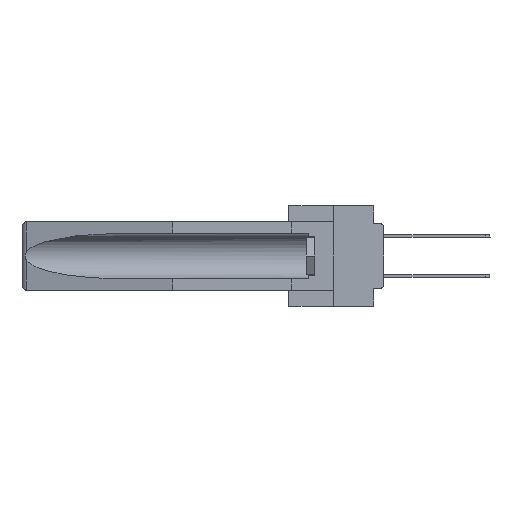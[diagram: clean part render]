
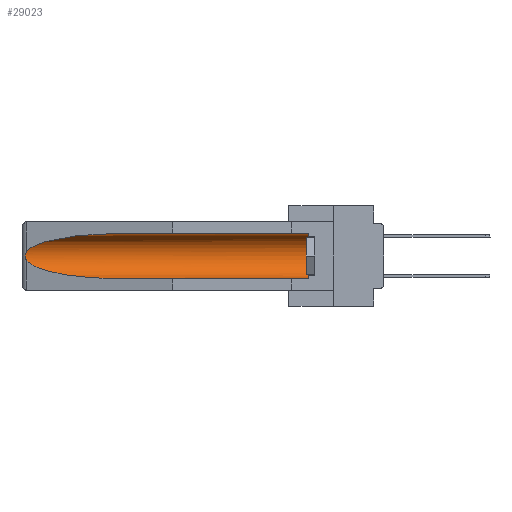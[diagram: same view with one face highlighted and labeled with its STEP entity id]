
A CAD part, left-side view. The second image highlights one B-rep face of the part: STEP entity #29023.
In plain terms, the highlighted cylindrical face has radius 2.857 mm (diameter 5.715 mm), a partial arc.
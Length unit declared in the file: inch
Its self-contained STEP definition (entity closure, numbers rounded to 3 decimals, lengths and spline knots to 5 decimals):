
#62 = VERTEX_POINT ( 'NONE', #29465 ) ;
#716 = VERTEX_POINT ( 'NONE', #33542 ) ;
#1018 = EDGE_CURVE ( 'NONE', #13209, #716, #25062, .T. ) ;
#1942 = CARTESIAN_POINT ( 'NONE',  ( 0.26655, 1.53094, -0.18657 ) ) ;
#3272 = VERTEX_POINT ( 'NONE', #4410 ) ;
#3542 = DIRECTION ( 'NONE',  ( 0., 0., 1. ) ) ;
#4410 = CARTESIAN_POINT ( 'NONE',  ( 0.155, 1.07973, -0.059 ) ) ;
#4457 = CARTESIAN_POINT ( 'NONE',  ( 0.26537, 1.52718, -0.14972 ) ) ;
#4753 = EDGE_CURVE ( 'NONE', #25559, #62, #9457, .T. ) ;
#5675 = VECTOR ( 'NONE', #8617, 39.37008 ) ;
#5806 = CARTESIAN_POINT ( 'NONE',  ( 0.26537, 1.52718, -0.19328 ) ) ;
#6232 = VERTEX_POINT ( 'NONE', #4457 ) ;
#7209 = CARTESIAN_POINT ( 'NONE',  ( 0.155, -0.30754, -0.284 ) ) ;
#8341 = CARTESIAN_POINT ( 'NONE',  ( 0.26537, 1.52718, -0.19328 ) ) ;
#8617 = DIRECTION ( 'NONE',  ( 0., 1., 0. ) ) ;
#9457 =( BOUNDED_CURVE ( )  B_SPLINE_CURVE ( 3, ( #8341, #11191, #31682, #26086 ),
 .UNSPECIFIED., .F., .F. ) 
 B_SPLINE_CURVE_WITH_KNOTS ( ( 4, 4 ),
 ( 0.1948, 1.5708 ),
 .UNSPECIFIED. ) 
 CURVE ( )  GEOMETRIC_REPRESENTATION_ITEM ( )  RATIONAL_B_SPLINE_CURVE ( ( 1., 0.848, 0.848, 1. ) ) 
 REPRESENTATION_ITEM ( '' )  );
#10147 = DIRECTION ( 'NONE',  ( 0., 1., 0. ) ) ;
#11191 = CARTESIAN_POINT ( 'NONE',  ( 0.25451, 1.48313, -0.24835 ) ) ;
#11286 = FACE_OUTER_BOUND ( 'NONE', #17979, .T. ) ;
#12970 = CARTESIAN_POINT ( 'NONE',  ( 0.26537, 1.52718, -0.14972 ) ) ;
#13188 = LINE ( 'NONE', #31208, #5675 ) ;
#13209 = VERTEX_POINT ( 'NONE', #27092 ) ;
#14999 = CARTESIAN_POINT ( 'NONE',  ( 0.25451, 1.48313, -0.09465 ) ) ;
#15819 = CARTESIAN_POINT ( 'NONE',  ( 0.26597, 1.5296, -0.19026 ) ) ;
#17310 = AXIS2_PLACEMENT_3D ( 'NONE', #30709, #36293, #33203 ) ;
#17743 = CARTESIAN_POINT ( 'NONE',  ( 0.21114, 1.30732, -0.059 ) ) ;
#17979 = EDGE_LOOP ( 'NONE', ( #22345, #20444, #34820, #32596, #23585, #20819 ) ) ;
#18168 = CARTESIAN_POINT ( 'NONE',  ( 0.155, -0.30754, -0.1715 ) ) ;
#18335 = EDGE_CURVE ( 'NONE', #6232, #25559, #19946, .T. ) ;
#19946 = B_SPLINE_CURVE_WITH_KNOTS ( 'NONE', 3,
 ( #12970, #29961, #24769, #35900, #32813, #21657, #21889, #1942, #15819, #27361 ),
 .UNSPECIFIED., .F., .F.,
 ( 4, 2, 2, 2, 4 ),
 ( 0., 0.00029, 0.00058, 0.00087, 0.00117 ),
 .UNSPECIFIED. ) ;
#20381 = EDGE_CURVE ( 'NONE', #716, #3272, #13188, .T. ) ;
#20444 = ORIENTED_EDGE ( 'NONE', *, *, #18335, .T. ) ;
#20819 = ORIENTED_EDGE ( 'NONE', *, *, #20381, .T. ) ;
#21657 = CARTESIAN_POINT ( 'NONE',  ( 0.2675, 1.53308, -0.17534 ) ) ;
#21889 = CARTESIAN_POINT ( 'NONE',  ( 0.2673, 1.53269, -0.17917 ) ) ;
#22345 = ORIENTED_EDGE ( 'NONE', *, *, #33107, .T. ) ;
#23585 = ORIENTED_EDGE ( 'NONE', *, *, #1018, .T. ) ;
#23983 = LINE ( 'NONE', #7209, #24884 ) ;
#24769 = CARTESIAN_POINT ( 'NONE',  ( 0.26654, 1.53092, -0.15636 ) ) ;
#24884 = VECTOR ( 'NONE', #10147, 39.37008 ) ;
#25062 = CIRCLE ( 'NONE', #17310, 0.1125 ) ;
#25559 = VERTEX_POINT ( 'NONE', #5806 ) ;
#26071 =( BOUNDED_CURVE ( )  B_SPLINE_CURVE ( 3, ( #32142, #17743, #14999, #34975 ),
 .UNSPECIFIED., .F., .T. ) 
 B_SPLINE_CURVE_WITH_KNOTS ( ( 4, 4 ),
 ( 4.71239, 6.08839 ),
 .UNSPECIFIED. ) 
 CURVE ( )  GEOMETRIC_REPRESENTATION_ITEM ( )  RATIONAL_B_SPLINE_CURVE ( ( 1., 0.848, 0.848, 1. ) ) 
 REPRESENTATION_ITEM ( '' )  );
#26086 = CARTESIAN_POINT ( 'NONE',  ( 0.155, 1.07973, -0.284 ) ) ;
#26389 = CYLINDRICAL_SURFACE ( 'NONE', #30545, 0.1125 ) ;
#27092 = CARTESIAN_POINT ( 'NONE',  ( 0.155, 0.126, -0.284 ) ) ;
#27361 = CARTESIAN_POINT ( 'NONE',  ( 0.26537, 1.52718, -0.19328 ) ) ;
#27842 = EDGE_CURVE ( 'NONE', #13209, #62, #23983, .T. ) ;
#29023 = ADVANCED_FACE ( 'NONE', ( #11286 ), #26389, .F. ) ;
#29205 = DIRECTION ( 'NONE',  ( 0., 1., 0. ) ) ;
#29465 = CARTESIAN_POINT ( 'NONE',  ( 0.155, 1.07973, -0.284 ) ) ;
#29961 = CARTESIAN_POINT ( 'NONE',  ( 0.26597, 1.52961, -0.15275 ) ) ;
#30545 = AXIS2_PLACEMENT_3D ( 'NONE', #18168, #29205, #3542 ) ;
#30709 = CARTESIAN_POINT ( 'NONE',  ( 0.155, 0.126, -0.1715 ) ) ;
#31208 = CARTESIAN_POINT ( 'NONE',  ( 0.155, -0.30754, -0.059 ) ) ;
#31682 = CARTESIAN_POINT ( 'NONE',  ( 0.21114, 1.30732, -0.284 ) ) ;
#32142 = CARTESIAN_POINT ( 'NONE',  ( 0.155, 1.07973, -0.059 ) ) ;
#32596 = ORIENTED_EDGE ( 'NONE', *, *, #27842, .F. ) ;
#32813 = CARTESIAN_POINT ( 'NONE',  ( 0.2675, 1.53308, -0.16763 ) ) ;
#33107 = EDGE_CURVE ( 'NONE', #3272, #6232, #26071, .T. ) ;
#33203 = DIRECTION ( 'NONE',  ( 0., 0., 1. ) ) ;
#33542 = CARTESIAN_POINT ( 'NONE',  ( 0.155, 0.126, -0.059 ) ) ;
#34820 = ORIENTED_EDGE ( 'NONE', *, *, #4753, .T. ) ;
#34975 = CARTESIAN_POINT ( 'NONE',  ( 0.26537, 1.52718, -0.14972 ) ) ;
#35900 = CARTESIAN_POINT ( 'NONE',  ( 0.2673, 1.5327, -0.16383 ) ) ;
#36293 = DIRECTION ( 'NONE',  ( 0., -1., 0. ) ) ;
